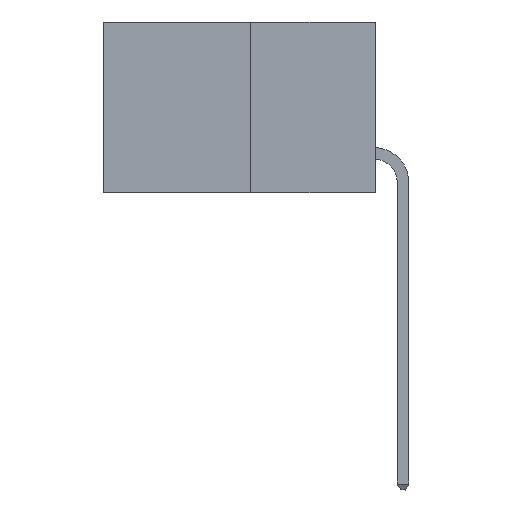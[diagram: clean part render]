
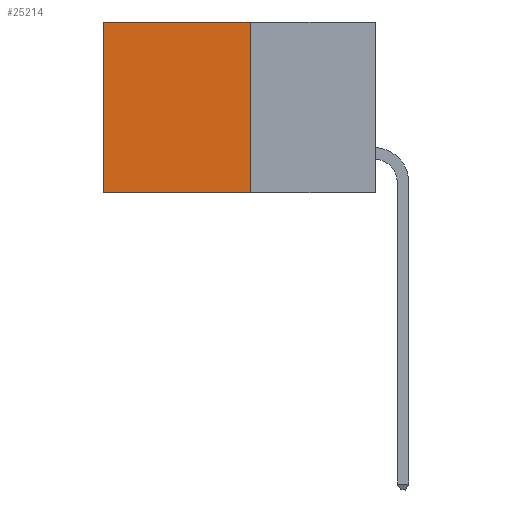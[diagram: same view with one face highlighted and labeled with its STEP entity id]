
A CAD part, left-side view. The second image highlights one B-rep face of the part: STEP entity #25214.
In plain terms, the highlighted planar face has unit normal (-1, 0, 0).
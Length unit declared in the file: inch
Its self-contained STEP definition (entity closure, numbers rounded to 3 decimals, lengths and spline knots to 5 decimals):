
#280 = CARTESIAN_POINT ( 'NONE',  ( 0.277, 0.59, -0.37 ) ) ;
#1015 = DIRECTION ( 'NONE',  ( 0., 0., -1. ) ) ;
#2115 = EDGE_CURVE ( 'NONE', #23919, #4510, #23929, .T. ) ;
#2738 = VECTOR ( 'NONE', #12002, 39.37008 ) ;
#3425 = LINE ( 'NONE', #20719, #2738 ) ;
#4294 = DIRECTION ( 'NONE',  ( 1., 0., 0. ) ) ;
#4510 = VERTEX_POINT ( 'NONE', #280 ) ;
#5487 = LINE ( 'NONE', #13068, #22130 ) ;
#8315 = EDGE_CURVE ( 'NONE', #23066, #4510, #5487, .T. ) ;
#10299 = AXIS2_PLACEMENT_3D ( 'NONE', #17294, #4294, #19503 ) ;
#10788 = ORIENTED_EDGE ( 'NONE', *, *, #21153, .F. ) ;
#12002 = DIRECTION ( 'NONE',  ( 0., 1., 0. ) ) ;
#12324 = CARTESIAN_POINT ( 'NONE',  ( 0.277, 0.27, 0. ) ) ;
#13068 = CARTESIAN_POINT ( 'NONE',  ( 0.277, 0.59, -0.37 ) ) ;
#13101 = LINE ( 'NONE', #26952, #18219 ) ;
#14021 = ORIENTED_EDGE ( 'NONE', *, *, #2115, .F. ) ;
#17294 = CARTESIAN_POINT ( 'NONE',  ( 0.277, 0.27, -0.37 ) ) ;
#18166 = VECTOR ( 'NONE', #22545, 39.37008 ) ;
#18219 = VECTOR ( 'NONE', #1015, 39.37008 ) ;
#18249 = ORIENTED_EDGE ( 'NONE', *, *, #23615, .T. ) ;
#18433 = CARTESIAN_POINT ( 'NONE',  ( 0.277, 0.59, 0. ) ) ;
#19503 = DIRECTION ( 'NONE',  ( 0., 0., -1. ) ) ;
#19572 = CARTESIAN_POINT ( 'NONE',  ( 0.277, 0.27, -0.37 ) ) ;
#19710 = FACE_OUTER_BOUND ( 'NONE', #27286, .T. ) ;
#19813 = ORIENTED_EDGE ( 'NONE', *, *, #8315, .T. ) ;
#20719 = CARTESIAN_POINT ( 'NONE',  ( 0.277, 0.27, 0. ) ) ;
#21153 = EDGE_CURVE ( 'NONE', #25038, #23919, #13101, .T. ) ;
#21934 = DIRECTION ( 'NONE',  ( 0., 0., -1. ) ) ;
#22130 = VECTOR ( 'NONE', #21934, 39.37008 ) ;
#22485 = CARTESIAN_POINT ( 'NONE',  ( 0.277, 0.27, -0.37 ) ) ;
#22545 = DIRECTION ( 'NONE',  ( 0., 1., 0. ) ) ;
#23066 = VERTEX_POINT ( 'NONE', #18433 ) ;
#23615 = EDGE_CURVE ( 'NONE', #25038, #23066, #3425, .T. ) ;
#23919 = VERTEX_POINT ( 'NONE', #19572 ) ;
#23929 = LINE ( 'NONE', #22485, #18166 ) ;
#25038 = VERTEX_POINT ( 'NONE', #12324 ) ;
#25214 = ADVANCED_FACE ( 'NONE', ( #19710 ), #27967, .F. ) ;
#26952 = CARTESIAN_POINT ( 'NONE',  ( 0.277, 0.27, -0.37 ) ) ;
#27286 = EDGE_LOOP ( 'NONE', ( #19813, #14021, #10788, #18249 ) ) ;
#27967 = PLANE ( 'NONE',  #10299 ) ;
